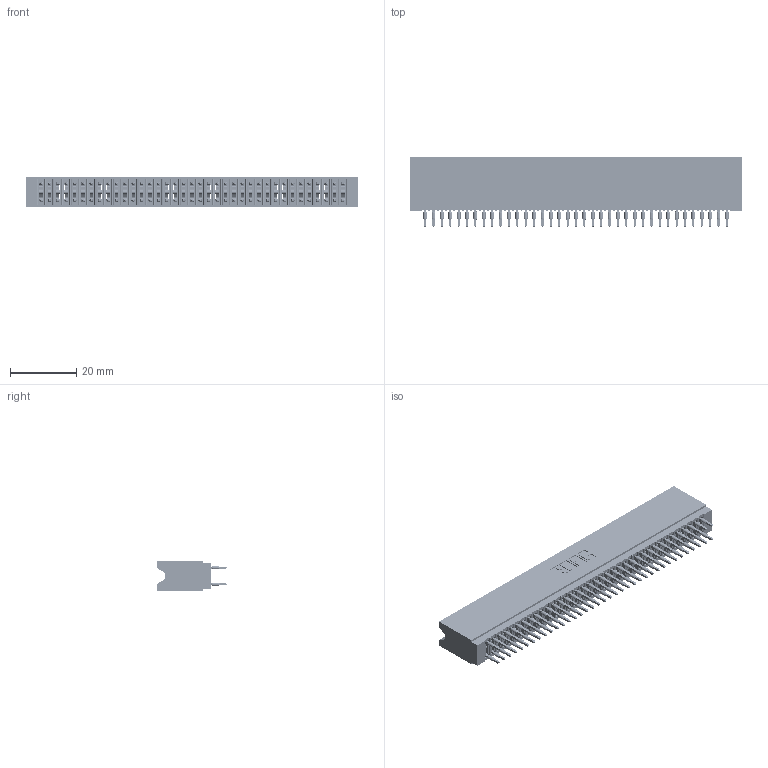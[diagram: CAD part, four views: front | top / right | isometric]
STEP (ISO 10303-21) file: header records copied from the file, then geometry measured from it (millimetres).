
FILE_DESCRIPTION (( 'STEP AP203' ), '1' );
FILE_NAME ('745-074-560-206.STEP', '2026-02-26T20:09:18', ( '' ), ( '' ), 'SwSTEP 2.0', 'SolidWorks 2023', '' );
FILE_SCHEMA (( 'CONFIG_CONTROL_DESIGN' ));
Length unit declared in the file: millimetre
Products named in the file (3): 745-074-560-206; 745-292-001_560; 745 Part_Insulator Option - 06
Assembly tree (75 placements, depth 2):
  745-074-560-206
    745 Part_Insulator Option - 06
    745-292-001_560  x74
Bounding box: 100.58 x 21.22 x 8.89 mm (x, y, z)
Volume: 9339.7 mm3; surface area: 20065.8 mm2
Topology: 75 solids, 75 shells, 7385 faces, 20203 edges, 12826 vertices
Faces by surface type: plane 3830, cylinder 1631, bspline 1480, torus 444
Entity records: 63316 total; most frequent: CARTESIAN_POINT 11488, ORIENTED_EDGE 10914, DIRECTION 9543, EDGE_CURVE 5457, LINE 5045, VECTOR 5045, VERTEX_POINT 3482, AXIS2_PLACEMENT_3D 2249
